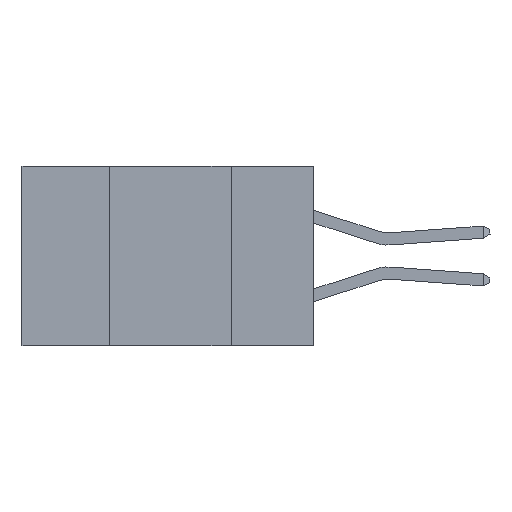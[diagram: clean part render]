
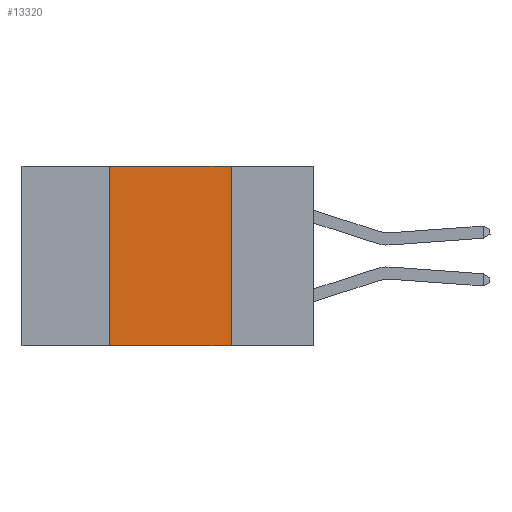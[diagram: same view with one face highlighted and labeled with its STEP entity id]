
A CAD part, left-side view. The second image highlights one B-rep face of the part: STEP entity #13320.
In plain terms, the highlighted planar face has unit normal (-1, 0, 0).
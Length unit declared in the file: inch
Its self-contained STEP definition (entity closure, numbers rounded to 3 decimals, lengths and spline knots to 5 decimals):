
#584 = CARTESIAN_POINT ( 'NONE',  ( 0., 0.17, -0.37 ) ) ;
#1450 = EDGE_CURVE ( 'NONE', #5084, #4107, #3398, .T. ) ;
#2020 = VECTOR ( 'NONE', #11689, 39.37008 ) ;
#2095 = LINE ( 'NONE', #10921, #5159 ) ;
#2559 = VERTEX_POINT ( 'NONE', #13221 ) ;
#2714 = EDGE_CURVE ( 'NONE', #2559, #4107, #8751, .T. ) ;
#2884 = CARTESIAN_POINT ( 'NONE',  ( 0., 0.6, 0. ) ) ;
#3398 = LINE ( 'NONE', #13058, #9590 ) ;
#4107 = VERTEX_POINT ( 'NONE', #584 ) ;
#4200 = DIRECTION ( 'NONE',  ( 0., 0., -1. ) ) ;
#4711 = AXIS2_PLACEMENT_3D ( 'NONE', #2884, #11491, #4200 ) ;
#5084 = VERTEX_POINT ( 'NONE', #7661 ) ;
#5159 = VECTOR ( 'NONE', #12132, 39.37008 ) ;
#7027 = VERTEX_POINT ( 'NONE', #10381 ) ;
#7344 = EDGE_CURVE ( 'NONE', #7027, #5084, #2095, .T. ) ;
#7406 = LINE ( 'NONE', #12323, #13066 ) ;
#7661 = CARTESIAN_POINT ( 'NONE',  ( 0., 0.17, 0. ) ) ;
#8748 = ORIENTED_EDGE ( 'NONE', *, *, #9420, .F. ) ;
#8751 = LINE ( 'NONE', #10243, #2020 ) ;
#9094 = PLANE ( 'NONE',  #4711 ) ;
#9420 = EDGE_CURVE ( 'NONE', #2559, #7027, #7406, .T. ) ;
#9468 = EDGE_LOOP ( 'NONE', ( #10087, #10448, #8748, #15155 ) ) ;
#9590 = VECTOR ( 'NONE', #12921, 39.37008 ) ;
#10087 = ORIENTED_EDGE ( 'NONE', *, *, #1450, .F. ) ;
#10133 = FACE_OUTER_BOUND ( 'NONE', #9468, .T. ) ;
#10243 = CARTESIAN_POINT ( 'NONE',  ( 0., 0.6, -0.37 ) ) ;
#10381 = CARTESIAN_POINT ( 'NONE',  ( 0., 0.42, 0. ) ) ;
#10448 = ORIENTED_EDGE ( 'NONE', *, *, #7344, .F. ) ;
#10921 = CARTESIAN_POINT ( 'NONE',  ( 0., 0.6, 0. ) ) ;
#11491 = DIRECTION ( 'NONE',  ( 1., 0., 0. ) ) ;
#11689 = DIRECTION ( 'NONE',  ( 0., -1., 0. ) ) ;
#12132 = DIRECTION ( 'NONE',  ( 0., -1., 0. ) ) ;
#12323 = CARTESIAN_POINT ( 'NONE',  ( 0., 0.42, 0. ) ) ;
#12921 = DIRECTION ( 'NONE',  ( 0., 0., -1. ) ) ;
#13058 = CARTESIAN_POINT ( 'NONE',  ( 0., 0.17, 0. ) ) ;
#13066 = VECTOR ( 'NONE', #14723, 39.37008 ) ;
#13221 = CARTESIAN_POINT ( 'NONE',  ( 0., 0.42, -0.37 ) ) ;
#13320 = ADVANCED_FACE ( 'NONE', ( #10133 ), #9094, .F. ) ;
#14723 = DIRECTION ( 'NONE',  ( 0., 0., 1. ) ) ;
#15155 = ORIENTED_EDGE ( 'NONE', *, *, #2714, .T. ) ;
